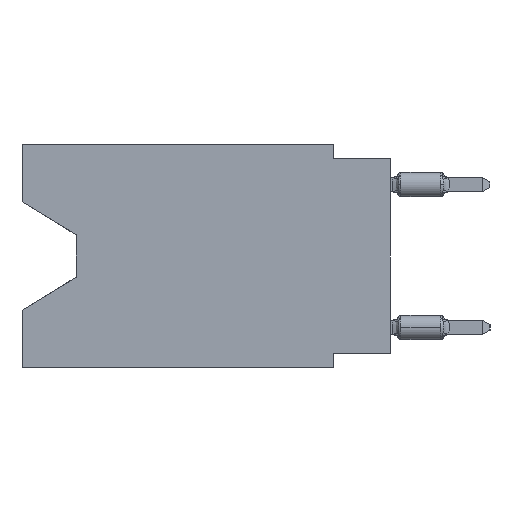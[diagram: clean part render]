
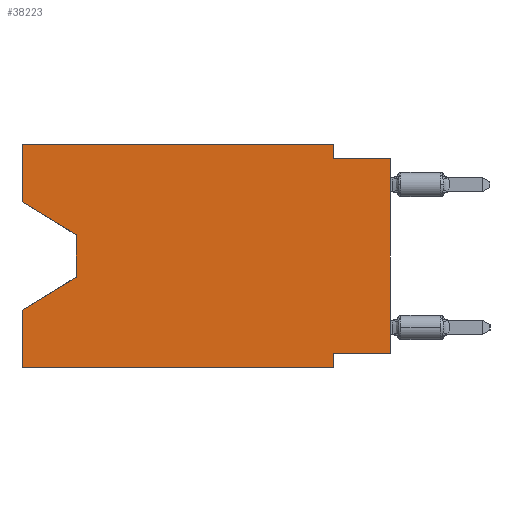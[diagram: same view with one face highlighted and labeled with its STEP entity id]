
A CAD part, left-side view. The second image highlights one B-rep face of the part: STEP entity #38223.
In plain terms, the highlighted planar face has unit normal (-1, 0, 0).
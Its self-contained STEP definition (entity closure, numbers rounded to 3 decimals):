
#942 = VECTOR ( 'NONE', #28976, 1000. ) ;
#1220 = LINE ( 'NONE', #7869, #39710 ) ;
#1877 = CARTESIAN_POINT ( 'NONE',  ( 0., 13.97, -5.893 ) ) ;
#2631 = CARTESIAN_POINT ( 'NONE',  ( 0., 13.97, -5.893 ) ) ;
#3031 = CARTESIAN_POINT ( 'NONE',  ( 0., 16.383, 0. ) ) ;
#3121 = AXIS2_PLACEMENT_3D ( 'NONE', #29704, #13434, #23426 ) ;
#3319 = CARTESIAN_POINT ( 'NONE',  ( 0., 2.54, 0. ) ) ;
#3709 = VECTOR ( 'NONE', #17942, 1000. ) ;
#4672 = CARTESIAN_POINT ( 'NONE',  ( 0., 16.383, 0. ) ) ;
#5601 = DIRECTION ( 'NONE',  ( 0., 0., -1. ) ) ;
#5753 = DIRECTION ( 'NONE',  ( 0., 0.855, -0.519 ) ) ;
#5850 = VERTEX_POINT ( 'NONE', #41139 ) ;
#6162 = CARTESIAN_POINT ( 'NONE',  ( 0., 16.383, -9.906 ) ) ;
#6451 = ORIENTED_EDGE ( 'NONE', *, *, #19603, .F. ) ;
#6986 = FACE_OUTER_BOUND ( 'NONE', #23761, .T. ) ;
#7063 = EDGE_CURVE ( 'NONE', #12910, #39599, #9272, .T. ) ;
#7092 = DIRECTION ( 'NONE',  ( 0., 0., -1. ) ) ;
#7506 = LINE ( 'NONE', #32953, #32096 ) ;
#7674 = ORIENTED_EDGE ( 'NONE', *, *, #13287, .F. ) ;
#7869 = CARTESIAN_POINT ( 'NONE',  ( 0., 16.383, -2.546 ) ) ;
#8168 = CARTESIAN_POINT ( 'NONE',  ( 0., 16.383, -2.546 ) ) ;
#8340 = DIRECTION ( 'NONE',  ( 0., 0., -1. ) ) ;
#8750 = CARTESIAN_POINT ( 'NONE',  ( 0., 2.54, -9.906 ) ) ;
#9111 = VERTEX_POINT ( 'NONE', #29282 ) ;
#9272 = LINE ( 'NONE', #3031, #26783 ) ;
#11466 = EDGE_CURVE ( 'NONE', #39947, #5850, #31436, .T. ) ;
#11609 = ORIENTED_EDGE ( 'NONE', *, *, #21273, .T. ) ;
#12152 = CARTESIAN_POINT ( 'NONE',  ( 0., 0., 0. ) ) ;
#12243 = LINE ( 'NONE', #30627, #12373 ) ;
#12373 = VECTOR ( 'NONE', #5601, 1000. ) ;
#12610 = LINE ( 'NONE', #6162, #33059 ) ;
#12903 = ORIENTED_EDGE ( 'NONE', *, *, #21931, .T. ) ;
#12910 = VERTEX_POINT ( 'NONE', #31364 ) ;
#12938 = VECTOR ( 'NONE', #8340, 1000. ) ;
#13065 = VECTOR ( 'NONE', #34765, 1000. ) ;
#13287 = EDGE_CURVE ( 'NONE', #33257, #26797, #38367, .T. ) ;
#13414 = ORIENTED_EDGE ( 'NONE', *, *, #17468, .T. ) ;
#13434 = DIRECTION ( 'NONE',  ( 1., 0., 0. ) ) ;
#14513 = DIRECTION ( 'NONE',  ( 0., -0.855, -0.519 ) ) ;
#14542 = ORIENTED_EDGE ( 'NONE', *, *, #37511, .F. ) ;
#16640 = VERTEX_POINT ( 'NONE', #28168 ) ;
#17468 = EDGE_CURVE ( 'NONE', #39947, #9111, #40741, .T. ) ;
#17942 = DIRECTION ( 'NONE',  ( 0., -1., 0. ) ) ;
#18668 = VERTEX_POINT ( 'NONE', #29370 ) ;
#19156 = CARTESIAN_POINT ( 'NONE',  ( 0., 16.383, 0. ) ) ;
#19603 = EDGE_CURVE ( 'NONE', #5850, #18668, #27929, .T. ) ;
#19605 = ORIENTED_EDGE ( 'NONE', *, *, #27647, .F. ) ;
#19993 = VECTOR ( 'NONE', #7092, 1000. ) ;
#20294 = PLANE ( 'NONE',  #3121 ) ;
#21073 = CARTESIAN_POINT ( 'NONE',  ( 0., 0., -0.635 ) ) ;
#21273 = EDGE_CURVE ( 'NONE', #16640, #39848, #32329, .T. ) ;
#21931 = EDGE_CURVE ( 'NONE', #39848, #39599, #40984, .T. ) ;
#21981 = DIRECTION ( 'NONE',  ( 0., -1., 0. ) ) ;
#23426 = DIRECTION ( 'NONE',  ( 0., 0., -1. ) ) ;
#23761 = EDGE_LOOP ( 'NONE', ( #30392, #11609, #12903, #25257, #34097, #6451, #40135, #13414, #33264, #14542, #7674, #19605 ) ) ;
#24098 = EDGE_CURVE ( 'NONE', #39882, #9111, #40069, .T. ) ;
#24975 = CARTESIAN_POINT ( 'NONE',  ( 0., 0., -9.271 ) ) ;
#25257 = ORIENTED_EDGE ( 'NONE', *, *, #7063, .F. ) ;
#25347 = EDGE_CURVE ( 'NONE', #26065, #16640, #1220, .T. ) ;
#26065 = VERTEX_POINT ( 'NONE', #8168 ) ;
#26783 = VECTOR ( 'NONE', #28473, 1000. ) ;
#26797 = VERTEX_POINT ( 'NONE', #3319 ) ;
#26885 = CARTESIAN_POINT ( 'NONE',  ( 0., 2.54, -0.635 ) ) ;
#27375 = VECTOR ( 'NONE', #5753, 1000. ) ;
#27647 = EDGE_CURVE ( 'NONE', #26065, #33257, #7506, .T. ) ;
#27929 = LINE ( 'NONE', #8750, #12938 ) ;
#28168 = CARTESIAN_POINT ( 'NONE',  ( 0., 13.97, -4.013 ) ) ;
#28473 = DIRECTION ( 'NONE',  ( 0., 0., 1. ) ) ;
#28976 = DIRECTION ( 'NONE',  ( 0., -1., 0. ) ) ;
#29282 = CARTESIAN_POINT ( 'NONE',  ( 0., 0., -0.635 ) ) ;
#29370 = CARTESIAN_POINT ( 'NONE',  ( 0., 2.54, -9.906 ) ) ;
#29704 = CARTESIAN_POINT ( 'NONE',  ( 0., 16.383, 0. ) ) ;
#30392 = ORIENTED_EDGE ( 'NONE', *, *, #25347, .T. ) ;
#30627 = CARTESIAN_POINT ( 'NONE',  ( 0., 2.54, 0. ) ) ;
#31364 = CARTESIAN_POINT ( 'NONE',  ( 0., 16.383, -9.906 ) ) ;
#31436 = LINE ( 'NONE', #41030, #13065 ) ;
#32096 = VECTOR ( 'NONE', #39015, 1000. ) ;
#32182 = VECTOR ( 'NONE', #33869, 1000. ) ;
#32329 = LINE ( 'NONE', #38794, #19993 ) ;
#32953 = CARTESIAN_POINT ( 'NONE',  ( 0., 16.383, 0. ) ) ;
#33059 = VECTOR ( 'NONE', #21981, 1000. ) ;
#33257 = VERTEX_POINT ( 'NONE', #4672 ) ;
#33264 = ORIENTED_EDGE ( 'NONE', *, *, #24098, .F. ) ;
#33869 = DIRECTION ( 'NONE',  ( 0., 0., 1. ) ) ;
#34097 = ORIENTED_EDGE ( 'NONE', *, *, #38131, .T. ) ;
#34765 = DIRECTION ( 'NONE',  ( 0., 1., 0. ) ) ;
#37511 = EDGE_CURVE ( 'NONE', #26797, #39882, #12243, .T. ) ;
#38025 = CARTESIAN_POINT ( 'NONE',  ( 0., 16.383, -7.36 ) ) ;
#38131 = EDGE_CURVE ( 'NONE', #12910, #18668, #12610, .T. ) ;
#38223 = ADVANCED_FACE ( 'NONE', ( #6986 ), #20294, .F. ) ;
#38367 = LINE ( 'NONE', #19156, #942 ) ;
#38794 = CARTESIAN_POINT ( 'NONE',  ( 0., 13.97, -4.013 ) ) ;
#39015 = DIRECTION ( 'NONE',  ( 0., 0., 1. ) ) ;
#39599 = VERTEX_POINT ( 'NONE', #38025 ) ;
#39710 = VECTOR ( 'NONE', #14513, 1000. ) ;
#39848 = VERTEX_POINT ( 'NONE', #1877 ) ;
#39882 = VERTEX_POINT ( 'NONE', #26885 ) ;
#39947 = VERTEX_POINT ( 'NONE', #24975 ) ;
#40069 = LINE ( 'NONE', #21073, #3709 ) ;
#40135 = ORIENTED_EDGE ( 'NONE', *, *, #11466, .F. ) ;
#40741 = LINE ( 'NONE', #12152, #32182 ) ;
#40984 = LINE ( 'NONE', #2631, #27375 ) ;
#41030 = CARTESIAN_POINT ( 'NONE',  ( 0., 0., -9.271 ) ) ;
#41139 = CARTESIAN_POINT ( 'NONE',  ( 0., 2.54, -9.271 ) ) ;
